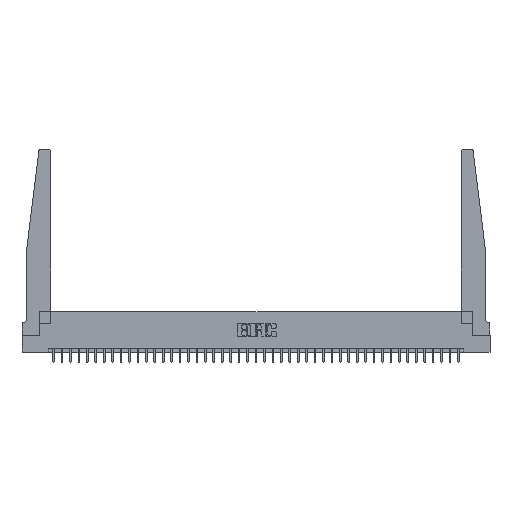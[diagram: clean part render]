
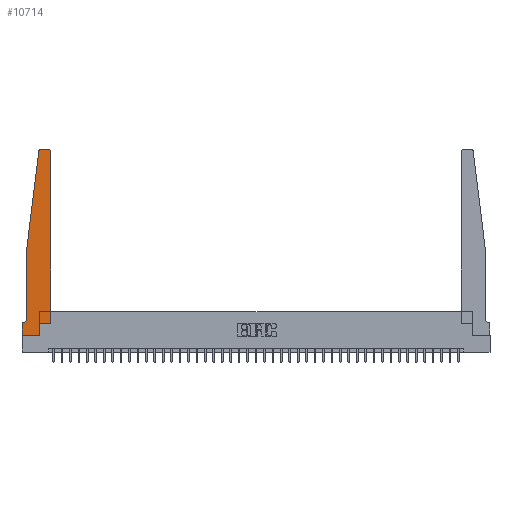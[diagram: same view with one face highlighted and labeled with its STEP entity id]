
A CAD part, top view. The second image highlights one B-rep face of the part: STEP entity #10714.
In plain terms, the highlighted planar face has unit normal (0, 0, 1).
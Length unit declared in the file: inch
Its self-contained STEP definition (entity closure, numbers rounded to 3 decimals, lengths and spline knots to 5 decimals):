
#106 = EDGE_LOOP ( 'NONE', ( #6772, #21282, #25324, #17929, #23746, #6133, #26841, #22016, #33614, #24855, #14035, #23028 ) ) ;
#1496 = VERTEX_POINT ( 'NONE', #23928 ) ;
#1537 = CARTESIAN_POINT ( 'NONE',  ( 0., 0., 0.37 ) ) ;
#2278 = LINE ( 'NONE', #2526, #16170 ) ;
#2526 = CARTESIAN_POINT ( 'NONE',  ( 0.065, 1.25, 0.37 ) ) ;
#3035 = VERTEX_POINT ( 'NONE', #1537 ) ;
#3265 = DIRECTION ( 'NONE',  ( 1., 0., 0. ) ) ;
#3325 = EDGE_CURVE ( 'NONE', #3035, #9547, #23832, .T. ) ;
#3402 = DIRECTION ( 'NONE',  ( 0., 0., 1. ) ) ;
#4216 = CARTESIAN_POINT ( 'NONE',  ( 0.395, 2.75, 0.37 ) ) ;
#4249 = EDGE_CURVE ( 'NONE', #1496, #14528, #19314, .T. ) ;
#4565 = EDGE_CURVE ( 'NONE', #13875, #12574, #31796, .T. ) ;
#4609 = CARTESIAN_POINT ( 'NONE',  ( 0.065, 0.2375, 0.37 ) ) ;
#4839 = DIRECTION ( 'NONE',  ( -0.122, -0.992, 0. ) ) ;
#5407 = CARTESIAN_POINT ( 'NONE',  ( 0.425, 0.18, 0.37 ) ) ;
#5543 = EDGE_CURVE ( 'NONE', #12574, #34135, #2278, .T. ) ;
#5848 = FACE_OUTER_BOUND ( 'NONE', #106, .T. ) ;
#6016 = CARTESIAN_POINT ( 'NONE',  ( 0., 0.1875, 0.37 ) ) ;
#6118 = DIRECTION ( 'NONE',  ( 0., 0., 1. ) ) ;
#6133 = ORIENTED_EDGE ( 'NONE', *, *, #14045, .T. ) ;
#6772 = ORIENTED_EDGE ( 'NONE', *, *, #14015, .T. ) ;
#7131 = VERTEX_POINT ( 'NONE', #10569 ) ;
#7564 = LINE ( 'NONE', #21616, #20642 ) ;
#8131 = EDGE_CURVE ( 'NONE', #30652, #1496, #11652, .T. ) ;
#8778 = AXIS2_PLACEMENT_3D ( 'NONE', #11757, #3402, #25449 ) ;
#9547 = VERTEX_POINT ( 'NONE', #31222 ) ;
#10569 = CARTESIAN_POINT ( 'NONE',  ( 0.015, 0.1875, 0.37 ) ) ;
#10714 = ADVANCED_FACE ( 'NONE', ( #5848 ), #19879, .T. ) ;
#11035 = AXIS2_PLACEMENT_3D ( 'NONE', #16339, #19242, #22269 ) ;
#11224 = CARTESIAN_POINT ( 'NONE',  ( 0.065, 1.25, 0.37 ) ) ;
#11652 = LINE ( 'NONE', #5407, #30226 ) ;
#11728 = VECTOR ( 'NONE', #27575, 39.37008 ) ;
#11757 = CARTESIAN_POINT ( 'NONE',  ( 0.27653, 2.72, 0.37 ) ) ;
#11851 = VECTOR ( 'NONE', #31084, 39.37008 ) ;
#12574 = VERTEX_POINT ( 'NONE', #14914 ) ;
#13566 = CARTESIAN_POINT ( 'NONE',  ( 0.2605, 0.18, 0.37 ) ) ;
#13808 = CARTESIAN_POINT ( 'NONE',  ( 0.015, 0.2375, 0.37 ) ) ;
#13875 = VERTEX_POINT ( 'NONE', #21399 ) ;
#14015 = EDGE_CURVE ( 'NONE', #14528, #13875, #30456, .T. ) ;
#14035 = ORIENTED_EDGE ( 'NONE', *, *, #8131, .T. ) ;
#14045 = EDGE_CURVE ( 'NONE', #7131, #15402, #19228, .T. ) ;
#14528 = VERTEX_POINT ( 'NONE', #4216 ) ;
#14914 = CARTESIAN_POINT ( 'NONE',  ( 0.24675, 2.72367, 0.37 ) ) ;
#14918 = VERTEX_POINT ( 'NONE', #4609 ) ;
#15145 = EDGE_CURVE ( 'NONE', #34135, #14918, #22592, .T. ) ;
#15402 = VERTEX_POINT ( 'NONE', #27891 ) ;
#16134 = DIRECTION ( 'NONE',  ( 1., 0., 0. ) ) ;
#16170 = VECTOR ( 'NONE', #4839, 39.37008 ) ;
#16339 = CARTESIAN_POINT ( 'NONE',  ( 0.395, 2.72, 0.37 ) ) ;
#16447 = VECTOR ( 'NONE', #25368, 39.37008 ) ;
#16547 = CARTESIAN_POINT ( 'NONE',  ( 0., 0., 0.37 ) ) ;
#16581 = DIRECTION ( 'NONE',  ( 0., 0., -1. ) ) ;
#16618 = VERTEX_POINT ( 'NONE', #28415 ) ;
#16713 = DIRECTION ( 'NONE',  ( 0., -1., 0. ) ) ;
#17261 = CARTESIAN_POINT ( 'NONE',  ( 0., 0., 0.37 ) ) ;
#17731 = DIRECTION ( 'NONE',  ( 0., -1., 0. ) ) ;
#17929 = ORIENTED_EDGE ( 'NONE', *, *, #15145, .T. ) ;
#18662 = LINE ( 'NONE', #13566, #11728 ) ;
#19228 = LINE ( 'NONE', #28181, #11851 ) ;
#19242 = DIRECTION ( 'NONE',  ( 0., 0., 1. ) ) ;
#19314 = CIRCLE ( 'NONE', #11035, 0.03 ) ;
#19879 = PLANE ( 'NONE',  #32524 ) ;
#20642 = VECTOR ( 'NONE', #16134, 39.37008 ) ;
#21042 = EDGE_CURVE ( 'NONE', #9547, #16618, #18662, .T. ) ;
#21282 = ORIENTED_EDGE ( 'NONE', *, *, #4565, .T. ) ;
#21399 = CARTESIAN_POINT ( 'NONE',  ( 0.27653, 2.75, 0.37 ) ) ;
#21616 = CARTESIAN_POINT ( 'NONE',  ( 0.425, 0.18, 0.37 ) ) ;
#22016 = ORIENTED_EDGE ( 'NONE', *, *, #3325, .T. ) ;
#22269 = DIRECTION ( 'NONE',  ( 1., 0., 0. ) ) ;
#22592 = LINE ( 'NONE', #11224, #23942 ) ;
#22835 = LINE ( 'NONE', #17261, #35373 ) ;
#23028 = ORIENTED_EDGE ( 'NONE', *, *, #4249, .T. ) ;
#23746 = ORIENTED_EDGE ( 'NONE', *, *, #32814, .T. ) ;
#23832 = LINE ( 'NONE', #16547, #16447 ) ;
#23928 = CARTESIAN_POINT ( 'NONE',  ( 0.425, 2.72, 0.37 ) ) ;
#23942 = VECTOR ( 'NONE', #16713, 39.37008 ) ;
#24802 = DIRECTION ( 'NONE',  ( 0., 1., 0. ) ) ;
#24855 = ORIENTED_EDGE ( 'NONE', *, *, #33690, .T. ) ;
#25324 = ORIENTED_EDGE ( 'NONE', *, *, #5543, .T. ) ;
#25368 = DIRECTION ( 'NONE',  ( 1., 0., 0. ) ) ;
#25449 = DIRECTION ( 'NONE',  ( 1., 0., 0. ) ) ;
#26841 = ORIENTED_EDGE ( 'NONE', *, *, #32157, .T. ) ;
#27575 = DIRECTION ( 'NONE',  ( 0., 1., 0. ) ) ;
#27891 = CARTESIAN_POINT ( 'NONE',  ( 0., 0.1875, 0.37 ) ) ;
#28181 = CARTESIAN_POINT ( 'NONE',  ( 0.065, 0.1875, 0.37 ) ) ;
#28415 = CARTESIAN_POINT ( 'NONE',  ( 0.2605, 0.18, 0.37 ) ) ;
#28511 = CARTESIAN_POINT ( 'NONE',  ( 0.065, 1.25, 0.37 ) ) ;
#30226 = VECTOR ( 'NONE', #24802, 39.37008 ) ;
#30456 = LINE ( 'NONE', #32831, #33492 ) ;
#30652 = VERTEX_POINT ( 'NONE', #31623 ) ;
#30725 = AXIS2_PLACEMENT_3D ( 'NONE', #13808, #16581, #32651 ) ;
#31084 = DIRECTION ( 'NONE',  ( -1., 0., 0. ) ) ;
#31222 = CARTESIAN_POINT ( 'NONE',  ( 0.2605, 0., 0.37 ) ) ;
#31623 = CARTESIAN_POINT ( 'NONE',  ( 0.425, 0.18, 0.37 ) ) ;
#31796 = CIRCLE ( 'NONE', #8778, 0.03 ) ;
#32157 = EDGE_CURVE ( 'NONE', #15402, #3035, #22835, .T. ) ;
#32524 = AXIS2_PLACEMENT_3D ( 'NONE', #6016, #6118, #3265 ) ;
#32651 = DIRECTION ( 'NONE',  ( -1., 0., 0. ) ) ;
#32814 = EDGE_CURVE ( 'NONE', #14918, #7131, #35790, .T. ) ;
#32831 = CARTESIAN_POINT ( 'NONE',  ( 0.25, 2.75, 0.37 ) ) ;
#33492 = VECTOR ( 'NONE', #35618, 39.37008 ) ;
#33614 = ORIENTED_EDGE ( 'NONE', *, *, #21042, .T. ) ;
#33690 = EDGE_CURVE ( 'NONE', #16618, #30652, #7564, .T. ) ;
#34135 = VERTEX_POINT ( 'NONE', #28511 ) ;
#35373 = VECTOR ( 'NONE', #17731, 39.37008 ) ;
#35618 = DIRECTION ( 'NONE',  ( -1., 0., 0. ) ) ;
#35790 = CIRCLE ( 'NONE', #30725, 0.05 ) ;
